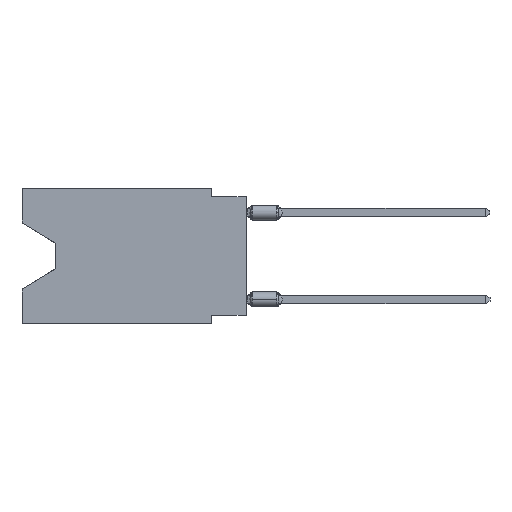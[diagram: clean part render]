
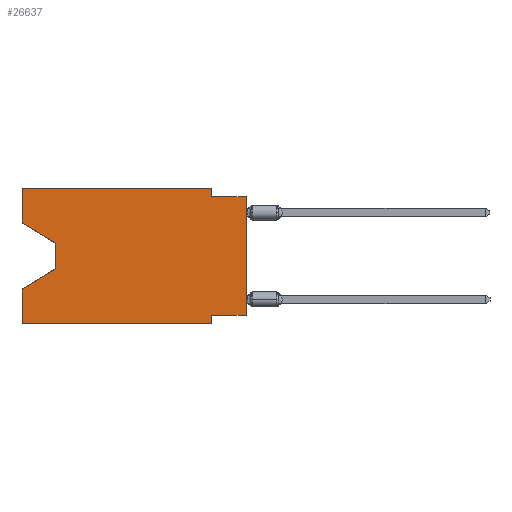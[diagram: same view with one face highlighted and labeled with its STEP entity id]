
A CAD part, left-side view. The second image highlights one B-rep face of the part: STEP entity #26637.
In plain terms, the highlighted planar face has unit normal (-1, 0, 0).
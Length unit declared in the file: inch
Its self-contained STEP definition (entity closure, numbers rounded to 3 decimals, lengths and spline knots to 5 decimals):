
#41 = PLANE ( 'NONE',  #20223 ) ;
#50 = LINE ( 'NONE', #6340, #21379 ) ;
#367 = CARTESIAN_POINT ( 'NONE',  ( 0., 0.645, 0. ) ) ;
#899 = ORIENTED_EDGE ( 'NONE', *, *, #25739, .T. ) ;
#1112 = VECTOR ( 'NONE', #21853, 39.37008 ) ;
#1165 = VERTEX_POINT ( 'NONE', #1739 ) ;
#1509 = VERTEX_POINT ( 'NONE', #1976 ) ;
#1517 = ORIENTED_EDGE ( 'NONE', *, *, #25287, .F. ) ;
#1605 = FACE_OUTER_BOUND ( 'NONE', #20732, .T. ) ;
#1739 = CARTESIAN_POINT ( 'NONE',  ( 0., 0.1, 0. ) ) ;
#1976 = CARTESIAN_POINT ( 'NONE',  ( 0., 0.55, -0.232 ) ) ;
#2383 = CARTESIAN_POINT ( 'NONE',  ( 0., 0.645, 0. ) ) ;
#2681 = VECTOR ( 'NONE', #7032, 39.37008 ) ;
#3467 = EDGE_CURVE ( 'NONE', #21062, #18368, #16229, .T. ) ;
#3780 = ORIENTED_EDGE ( 'NONE', *, *, #25628, .F. ) ;
#3862 = CARTESIAN_POINT ( 'NONE',  ( 0., 0.645, -0.28975 ) ) ;
#3879 = CARTESIAN_POINT ( 'NONE',  ( 0., 0.645, 0. ) ) ;
#4136 = CARTESIAN_POINT ( 'NONE',  ( 0., 0.645, -0.39 ) ) ;
#4252 = CARTESIAN_POINT ( 'NONE',  ( 0., 0.1, -0.39 ) ) ;
#4572 = EDGE_CURVE ( 'NONE', #13403, #8766, #8229, .T. ) ;
#4573 = DIRECTION ( 'NONE',  ( 0., 1., 0. ) ) ;
#4840 = CARTESIAN_POINT ( 'NONE',  ( 0., 0., -0.025 ) ) ;
#4988 = CARTESIAN_POINT ( 'NONE',  ( 0., 0.1, 0. ) ) ;
#5066 = ORIENTED_EDGE ( 'NONE', *, *, #18093, .T. ) ;
#5839 = DIRECTION ( 'NONE',  ( 0., 0., 1. ) ) ;
#6229 = VECTOR ( 'NONE', #19705, 39.37008 ) ;
#6340 = CARTESIAN_POINT ( 'NONE',  ( 0., 0., -0.365 ) ) ;
#7032 = DIRECTION ( 'NONE',  ( 0., 0.855, -0.519 ) ) ;
#7170 = DIRECTION ( 'NONE',  ( 0., 0., -1. ) ) ;
#7521 = ORIENTED_EDGE ( 'NONE', *, *, #3467, .F. ) ;
#7572 = DIRECTION ( 'NONE',  ( 0., -1., 0. ) ) ;
#7583 = VECTOR ( 'NONE', #7170, 39.37008 ) ;
#7702 = VERTEX_POINT ( 'NONE', #17173 ) ;
#7836 = LINE ( 'NONE', #3879, #21920 ) ;
#8229 = LINE ( 'NONE', #4136, #25801 ) ;
#8496 = VECTOR ( 'NONE', #20495, 39.37008 ) ;
#8626 = CARTESIAN_POINT ( 'NONE',  ( 0., 0.1, -0.365 ) ) ;
#8766 = VERTEX_POINT ( 'NONE', #4252 ) ;
#8785 = EDGE_CURVE ( 'NONE', #13566, #7702, #24769, .T. ) ;
#9169 = LINE ( 'NONE', #17502, #6229 ) ;
#9198 = ORIENTED_EDGE ( 'NONE', *, *, #16013, .F. ) ;
#9728 = EDGE_CURVE ( 'NONE', #13566, #11392, #50, .T. ) ;
#9849 = LINE ( 'NONE', #9984, #12321 ) ;
#9947 = VERTEX_POINT ( 'NONE', #3862 ) ;
#9984 = CARTESIAN_POINT ( 'NONE',  ( 0., 0.55, -0.158 ) ) ;
#10937 = VECTOR ( 'NONE', #12893, 39.37008 ) ;
#10996 = EDGE_CURVE ( 'NONE', #15149, #7702, #14825, .T. ) ;
#11074 = EDGE_CURVE ( 'NONE', #1509, #9947, #19865, .T. ) ;
#11079 = CARTESIAN_POINT ( 'NONE',  ( 0., 0.1, -0.025 ) ) ;
#11392 = VERTEX_POINT ( 'NONE', #8626 ) ;
#11707 = LINE ( 'NONE', #20048, #1112 ) ;
#12321 = VECTOR ( 'NONE', #17916, 39.37008 ) ;
#12432 = EDGE_CURVE ( 'NONE', #13403, #9947, #22080, .T. ) ;
#12893 = DIRECTION ( 'NONE',  ( 0., -1., 0. ) ) ;
#13403 = VERTEX_POINT ( 'NONE', #17557 ) ;
#13553 = CARTESIAN_POINT ( 'NONE',  ( 0., 0.645, -0.10025 ) ) ;
#13566 = VERTEX_POINT ( 'NONE', #18226 ) ;
#14318 = CARTESIAN_POINT ( 'NONE',  ( 0., 0.645, 0. ) ) ;
#14825 = LINE ( 'NONE', #4840, #10937 ) ;
#15149 = VERTEX_POINT ( 'NONE', #11079 ) ;
#16013 = EDGE_CURVE ( 'NONE', #1165, #15149, #23700, .T. ) ;
#16149 = VERTEX_POINT ( 'NONE', #26554 ) ;
#16229 = LINE ( 'NONE', #14318, #20030 ) ;
#16411 = CARTESIAN_POINT ( 'NONE',  ( 0., 0., 0. ) ) ;
#16861 = ORIENTED_EDGE ( 'NONE', *, *, #11074, .T. ) ;
#17173 = CARTESIAN_POINT ( 'NONE',  ( 0., 0., -0.025 ) ) ;
#17223 = DIRECTION ( 'NONE',  ( 0., -1., 0. ) ) ;
#17502 = CARTESIAN_POINT ( 'NONE',  ( 0., 0.1, -0.39 ) ) ;
#17557 = CARTESIAN_POINT ( 'NONE',  ( 0., 0.645, -0.39 ) ) ;
#17707 = DIRECTION ( 'NONE',  ( 0., 0., 1. ) ) ;
#17916 = DIRECTION ( 'NONE',  ( 0., 0., -1. ) ) ;
#18093 = EDGE_CURVE ( 'NONE', #21062, #16149, #11707, .T. ) ;
#18226 = CARTESIAN_POINT ( 'NONE',  ( 0., 0., -0.365 ) ) ;
#18368 = VERTEX_POINT ( 'NONE', #367 ) ;
#18755 = DIRECTION ( 'NONE',  ( 0., 0., -1. ) ) ;
#19705 = DIRECTION ( 'NONE',  ( 0., 0., -1. ) ) ;
#19716 = VECTOR ( 'NONE', #17707, 39.37008 ) ;
#19865 = LINE ( 'NONE', #24231, #2681 ) ;
#20030 = VECTOR ( 'NONE', #5839, 39.37008 ) ;
#20048 = CARTESIAN_POINT ( 'NONE',  ( 0., 0.645, -0.10025 ) ) ;
#20223 = AXIS2_PLACEMENT_3D ( 'NONE', #2383, #20812, #18755 ) ;
#20421 = CARTESIAN_POINT ( 'NONE',  ( 0., 0.645, 0. ) ) ;
#20495 = DIRECTION ( 'NONE',  ( 0., 0., 1. ) ) ;
#20732 = EDGE_LOOP ( 'NONE', ( #5066, #899, #16861, #22310, #25558, #3780, #24310, #25343, #20840, #9198, #1517, #7521 ) ) ;
#20812 = DIRECTION ( 'NONE',  ( 1., 0., 0. ) ) ;
#20840 = ORIENTED_EDGE ( 'NONE', *, *, #10996, .F. ) ;
#21062 = VERTEX_POINT ( 'NONE', #13553 ) ;
#21379 = VECTOR ( 'NONE', #4573, 39.37008 ) ;
#21853 = DIRECTION ( 'NONE',  ( 0., -0.855, -0.519 ) ) ;
#21920 = VECTOR ( 'NONE', #7572, 39.37008 ) ;
#22080 = LINE ( 'NONE', #20421, #19716 ) ;
#22310 = ORIENTED_EDGE ( 'NONE', *, *, #12432, .F. ) ;
#23700 = LINE ( 'NONE', #4988, #7583 ) ;
#24231 = CARTESIAN_POINT ( 'NONE',  ( 0., 0.55, -0.232 ) ) ;
#24310 = ORIENTED_EDGE ( 'NONE', *, *, #9728, .F. ) ;
#24769 = LINE ( 'NONE', #16411, #8496 ) ;
#25287 = EDGE_CURVE ( 'NONE', #18368, #1165, #7836, .T. ) ;
#25343 = ORIENTED_EDGE ( 'NONE', *, *, #8785, .T. ) ;
#25558 = ORIENTED_EDGE ( 'NONE', *, *, #4572, .T. ) ;
#25628 = EDGE_CURVE ( 'NONE', #11392, #8766, #9169, .T. ) ;
#25739 = EDGE_CURVE ( 'NONE', #16149, #1509, #9849, .T. ) ;
#25801 = VECTOR ( 'NONE', #17223, 39.37008 ) ;
#26554 = CARTESIAN_POINT ( 'NONE',  ( 0., 0.55, -0.158 ) ) ;
#26637 = ADVANCED_FACE ( 'NONE', ( #1605 ), #41, .F. ) ;
